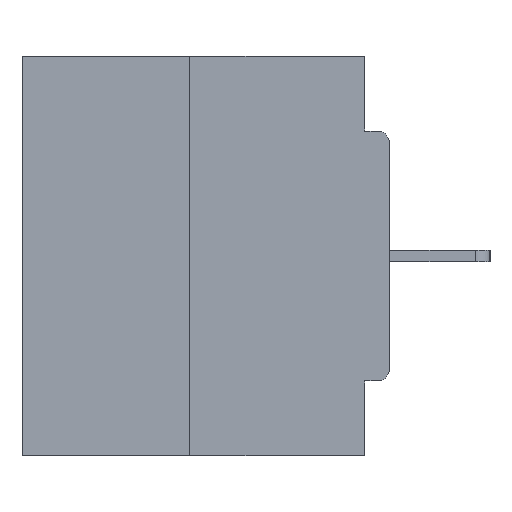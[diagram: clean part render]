
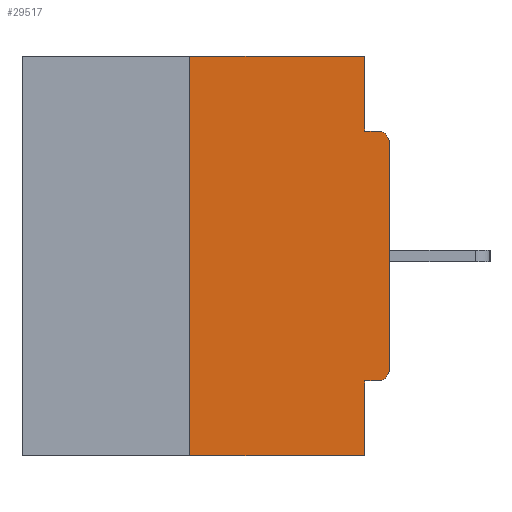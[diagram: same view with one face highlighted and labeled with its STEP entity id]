
A CAD part, left-side view. The second image highlights one B-rep face of the part: STEP entity #29517.
In plain terms, the highlighted planar face has unit normal (-1, 0, 0).
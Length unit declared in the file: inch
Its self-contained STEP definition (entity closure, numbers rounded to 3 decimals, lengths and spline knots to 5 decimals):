
#906 = CARTESIAN_POINT ( 'NONE',  ( 0., 0.25, 0. ) ) ;
#2591 = LINE ( 'NONE', #28541, #16491 ) ;
#2603 = VECTOR ( 'NONE', #29349, 39.37008 ) ;
#2759 = VERTEX_POINT ( 'NONE', #13902 ) ;
#3095 = DIRECTION ( 'NONE',  ( 0., -1., 0. ) ) ;
#3099 = CARTESIAN_POINT ( 'NONE',  ( 0., 0.015, -0.3915 ) ) ;
#3225 = VERTEX_POINT ( 'NONE', #9514 ) ;
#3752 = DIRECTION ( 'NONE',  ( 0., 0., -1. ) ) ;
#4816 = EDGE_CURVE ( 'NONE', #21024, #25820, #15118, .T. ) ;
#5122 = DIRECTION ( 'NONE',  ( 0., 0., -1. ) ) ;
#5661 = CARTESIAN_POINT ( 'NONE',  ( 0., 0.015, -0.4065 ) ) ;
#6274 = EDGE_CURVE ( 'NONE', #3225, #2759, #21130, .T. ) ;
#6394 = EDGE_CURVE ( 'NONE', #29212, #10008, #9492, .T. ) ;
#6782 = ORIENTED_EDGE ( 'NONE', *, *, #6394, .T. ) ;
#7438 = CARTESIAN_POINT ( 'NONE',  ( 0., 0.46, 0. ) ) ;
#7592 = DIRECTION ( 'NONE',  ( 0., 0., -1. ) ) ;
#8301 = VERTEX_POINT ( 'NONE', #22847 ) ;
#8677 = CARTESIAN_POINT ( 'NONE',  ( 0., 0.031, 0. ) ) ;
#8864 = CARTESIAN_POINT ( 'NONE',  ( 0., 0.015, -0.0935 ) ) ;
#9253 = VECTOR ( 'NONE', #26439, 39.37008 ) ;
#9492 = LINE ( 'NONE', #14619, #9253 ) ;
#9514 = CARTESIAN_POINT ( 'NONE',  ( 0., 0., -0.3915 ) ) ;
#9936 = DIRECTION ( 'NONE',  ( 1., 0., 0. ) ) ;
#10008 = VERTEX_POINT ( 'NONE', #20671 ) ;
#10200 = ORIENTED_EDGE ( 'NONE', *, *, #23878, .F. ) ;
#10240 = LINE ( 'NONE', #906, #2603 ) ;
#10914 = CARTESIAN_POINT ( 'NONE',  ( 0., 0.031, 0. ) ) ;
#11740 = VECTOR ( 'NONE', #30468, 39.37008 ) ;
#12172 = ORIENTED_EDGE ( 'NONE', *, *, #29242, .T. ) ;
#12265 = FACE_OUTER_BOUND ( 'NONE', #28406, .T. ) ;
#12398 = ORIENTED_EDGE ( 'NONE', *, *, #29856, .F. ) ;
#12912 = CARTESIAN_POINT ( 'NONE',  ( 0., 0.25, -0.5 ) ) ;
#12956 = ORIENTED_EDGE ( 'NONE', *, *, #27748, .F. ) ;
#12959 = ORIENTED_EDGE ( 'NONE', *, *, #29610, .F. ) ;
#13902 = CARTESIAN_POINT ( 'NONE',  ( 0., 0., -0.1085 ) ) ;
#14001 = LINE ( 'NONE', #28147, #26322 ) ;
#14619 = CARTESIAN_POINT ( 'NONE',  ( 0., 0.46, -0.5 ) ) ;
#14638 = ORIENTED_EDGE ( 'NONE', *, *, #4816, .F. ) ;
#15118 = LINE ( 'NONE', #10914, #17720 ) ;
#15384 = CARTESIAN_POINT ( 'NONE',  ( 0., 0.015, -0.1085 ) ) ;
#15488 = ORIENTED_EDGE ( 'NONE', *, *, #27582, .F. ) ;
#15959 = VERTEX_POINT ( 'NONE', #5661 ) ;
#16491 = VECTOR ( 'NONE', #21539, 39.37008 ) ;
#16983 = AXIS2_PLACEMENT_3D ( 'NONE', #3099, #24529, #7592 ) ;
#17399 = VECTOR ( 'NONE', #3095, 39.37008 ) ;
#17720 = VECTOR ( 'NONE', #3752, 39.37008 ) ;
#18520 = CARTESIAN_POINT ( 'NONE',  ( 0., 0.031, -0.0935 ) ) ;
#18582 = CARTESIAN_POINT ( 'NONE',  ( 0., 0.031, -0.5 ) ) ;
#20671 = CARTESIAN_POINT ( 'NONE',  ( 0., 0.031, -0.5 ) ) ;
#20934 = AXIS2_PLACEMENT_3D ( 'NONE', #15384, #22826, #25013 ) ;
#21024 = VERTEX_POINT ( 'NONE', #8677 ) ;
#21130 = LINE ( 'NONE', #30618, #11740 ) ;
#21201 = ORIENTED_EDGE ( 'NONE', *, *, #29551, .T. ) ;
#21539 = DIRECTION ( 'NONE',  ( 0., -1., 0. ) ) ;
#21823 = VERTEX_POINT ( 'NONE', #8864 ) ;
#22634 = LINE ( 'NONE', #24376, #17399 ) ;
#22826 = DIRECTION ( 'NONE',  ( -1., 0., 0. ) ) ;
#22847 = CARTESIAN_POINT ( 'NONE',  ( 0., 0.031, -0.4065 ) ) ;
#22929 = AXIS2_PLACEMENT_3D ( 'NONE', #7438, #9936, #5122 ) ;
#23467 = DIRECTION ( 'NONE',  ( 0., 1., 0. ) ) ;
#23798 = VERTEX_POINT ( 'NONE', #25907 ) ;
#23878 = EDGE_CURVE ( 'NONE', #25820, #21823, #2591, .T. ) ;
#24376 = CARTESIAN_POINT ( 'NONE',  ( 0., 0.46, 0. ) ) ;
#24529 = DIRECTION ( 'NONE',  ( -1., 0., 0. ) ) ;
#25013 = DIRECTION ( 'NONE',  ( 0., 0., -1. ) ) ;
#25426 = CIRCLE ( 'NONE', #16983, 0.015 ) ;
#25820 = VERTEX_POINT ( 'NONE', #18520 ) ;
#25907 = CARTESIAN_POINT ( 'NONE',  ( 0., 0.25, 0. ) ) ;
#26322 = VECTOR ( 'NONE', #23467, 39.37008 ) ;
#26439 = DIRECTION ( 'NONE',  ( 0., -1., 0. ) ) ;
#26856 = VECTOR ( 'NONE', #28078, 39.37008 ) ;
#27582 = EDGE_CURVE ( 'NONE', #23798, #21024, #22634, .T. ) ;
#27748 = EDGE_CURVE ( 'NONE', #15959, #8301, #14001, .T. ) ;
#28078 = DIRECTION ( 'NONE',  ( 0., 0., -1. ) ) ;
#28147 = CARTESIAN_POINT ( 'NONE',  ( 0., 0., -0.4065 ) ) ;
#28406 = EDGE_LOOP ( 'NONE', ( #15488, #12959, #6782, #12398, #12956, #21201, #28938, #12172, #10200, #14638 ) ) ;
#28541 = CARTESIAN_POINT ( 'NONE',  ( 0., 0., -0.0935 ) ) ;
#28723 = PLANE ( 'NONE',  #22929 ) ;
#28938 = ORIENTED_EDGE ( 'NONE', *, *, #6274, .T. ) ;
#29212 = VERTEX_POINT ( 'NONE', #12912 ) ;
#29242 = EDGE_CURVE ( 'NONE', #2759, #21823, #29408, .T. ) ;
#29349 = DIRECTION ( 'NONE',  ( 0., 0., 1. ) ) ;
#29408 = CIRCLE ( 'NONE', #20934, 0.015 ) ;
#29517 = ADVANCED_FACE ( 'NONE', ( #12265 ), #28723, .F. ) ;
#29551 = EDGE_CURVE ( 'NONE', #15959, #3225, #25426, .T. ) ;
#29610 = EDGE_CURVE ( 'NONE', #29212, #23798, #10240, .T. ) ;
#29856 = EDGE_CURVE ( 'NONE', #8301, #10008, #30410, .T. ) ;
#30410 = LINE ( 'NONE', #18582, #26856 ) ;
#30468 = DIRECTION ( 'NONE',  ( 0., 0., 1. ) ) ;
#30618 = CARTESIAN_POINT ( 'NONE',  ( 0., 0., 0. ) ) ;
